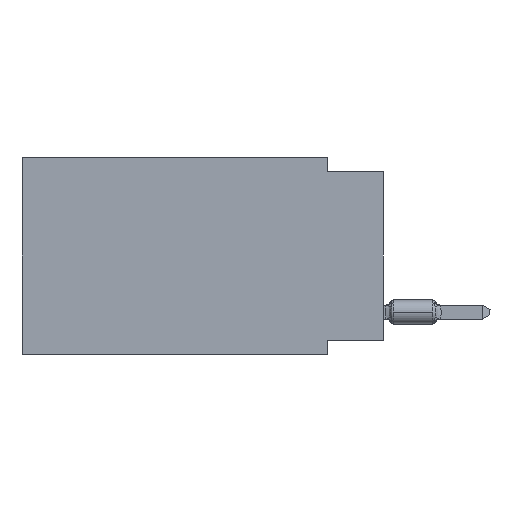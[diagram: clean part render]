
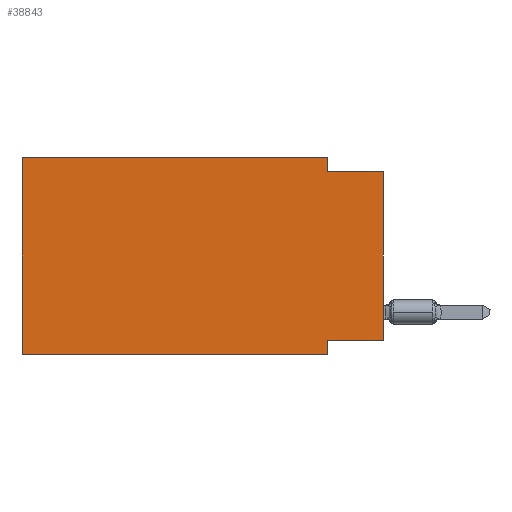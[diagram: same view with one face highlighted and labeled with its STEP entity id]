
A CAD part, left-side view. The second image highlights one B-rep face of the part: STEP entity #38843.
In plain terms, the highlighted planar face has unit normal (-1, 0, 0).
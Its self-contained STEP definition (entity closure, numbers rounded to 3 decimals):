
#959 = EDGE_CURVE ( 'NONE', #42400, #59429, #41404, .T. ) ;
#995 = CARTESIAN_POINT ( 'NONE',  ( 0., 2.54, 0. ) ) ;
#5017 = VECTOR ( 'NONE', #26155, 1000. ) ;
#5420 = VERTEX_POINT ( 'NONE', #23534 ) ;
#5710 = ORIENTED_EDGE ( 'NONE', *, *, #33910, .T. ) ;
#6240 = CARTESIAN_POINT ( 'NONE',  ( 0., 16.383, 0. ) ) ;
#8105 = VECTOR ( 'NONE', #15384, 1000. ) ;
#8938 = ORIENTED_EDGE ( 'NONE', *, *, #44442, .F. ) ;
#8968 = CARTESIAN_POINT ( 'NONE',  ( 0., 0., -8.255 ) ) ;
#9384 = LINE ( 'NONE', #24396, #17201 ) ;
#15384 = DIRECTION ( 'NONE',  ( 0., 0., -1. ) ) ;
#16372 = LINE ( 'NONE', #6240, #5017 ) ;
#17201 = VECTOR ( 'NONE', #40346, 1000. ) ;
#18650 = DIRECTION ( 'NONE',  ( 1., 0., 0. ) ) ;
#19373 = EDGE_CURVE ( 'NONE', #58460, #5420, #9384, .T. ) ;
#20087 = VECTOR ( 'NONE', #61291, 1000. ) ;
#20989 = CARTESIAN_POINT ( 'NONE',  ( 0., 2.54, -8.255 ) ) ;
#21630 = ORIENTED_EDGE ( 'NONE', *, *, #31650, .T. ) ;
#22171 = EDGE_CURVE ( 'NONE', #61417, #42400, #30371, .T. ) ;
#22909 = ORIENTED_EDGE ( 'NONE', *, *, #24747, .F. ) ;
#23534 = CARTESIAN_POINT ( 'NONE',  ( 0., 16.383, 0. ) ) ;
#24181 = VERTEX_POINT ( 'NONE', #8968 ) ;
#24396 = CARTESIAN_POINT ( 'NONE',  ( 0., 16.383, 0. ) ) ;
#24747 = EDGE_CURVE ( 'NONE', #5420, #61417, #16372, .T. ) ;
#25201 = CARTESIAN_POINT ( 'NONE',  ( 0., 16.383, -8.89 ) ) ;
#25413 = CARTESIAN_POINT ( 'NONE',  ( 0., 16.383, -8.89 ) ) ;
#25518 = DIRECTION ( 'NONE',  ( 0., -1., 0. ) ) ;
#26053 = LINE ( 'NONE', #27330, #51731 ) ;
#26155 = DIRECTION ( 'NONE',  ( 0., -1., 0. ) ) ;
#27330 = CARTESIAN_POINT ( 'NONE',  ( 0., 0., 0. ) ) ;
#27706 = CARTESIAN_POINT ( 'NONE',  ( 0., 2.54, 0. ) ) ;
#28099 = ORIENTED_EDGE ( 'NONE', *, *, #19373, .F. ) ;
#28389 = VERTEX_POINT ( 'NONE', #58267 ) ;
#28462 = DIRECTION ( 'NONE',  ( 0., 1., 0. ) ) ;
#29060 = PLANE ( 'NONE',  #57670 ) ;
#30371 = LINE ( 'NONE', #995, #8105 ) ;
#31650 = EDGE_CURVE ( 'NONE', #24181, #59429, #26053, .T. ) ;
#32051 = EDGE_LOOP ( 'NONE', ( #21630, #54140, #35988, #22909, #28099, #5710, #8938, #35703 ) ) ;
#32272 = CARTESIAN_POINT ( 'NONE',  ( 0., 0., -0.635 ) ) ;
#33348 = CARTESIAN_POINT ( 'NONE',  ( 0., 0., -8.255 ) ) ;
#33910 = EDGE_CURVE ( 'NONE', #58460, #28389, #34969, .T. ) ;
#34969 = LINE ( 'NONE', #25201, #51903 ) ;
#35703 = ORIENTED_EDGE ( 'NONE', *, *, #49704, .F. ) ;
#35988 = ORIENTED_EDGE ( 'NONE', *, *, #22171, .F. ) ;
#37371 = VECTOR ( 'NONE', #60316, 1000. ) ;
#37729 = CARTESIAN_POINT ( 'NONE',  ( 0., 0., -0.635 ) ) ;
#38843 = ADVANCED_FACE ( 'NONE', ( #58739 ), #29060, .F. ) ;
#40346 = DIRECTION ( 'NONE',  ( 0., 0., 1. ) ) ;
#41404 = LINE ( 'NONE', #32272, #20087 ) ;
#41704 = LINE ( 'NONE', #45985, #37371 ) ;
#42400 = VERTEX_POINT ( 'NONE', #47348 ) ;
#42772 = CARTESIAN_POINT ( 'NONE',  ( 0., 16.383, 0. ) ) ;
#44442 = EDGE_CURVE ( 'NONE', #60667, #28389, #41704, .T. ) ;
#45985 = CARTESIAN_POINT ( 'NONE',  ( 0., 2.54, -8.89 ) ) ;
#47348 = CARTESIAN_POINT ( 'NONE',  ( 0., 2.54, -0.635 ) ) ;
#49704 = EDGE_CURVE ( 'NONE', #24181, #60667, #53235, .T. ) ;
#51731 = VECTOR ( 'NONE', #56351, 1000. ) ;
#51903 = VECTOR ( 'NONE', #25518, 1000. ) ;
#53235 = LINE ( 'NONE', #33348, #53658 ) ;
#53658 = VECTOR ( 'NONE', #28462, 1000. ) ;
#54140 = ORIENTED_EDGE ( 'NONE', *, *, #959, .F. ) ;
#56351 = DIRECTION ( 'NONE',  ( 0., 0., 1. ) ) ;
#57670 = AXIS2_PLACEMENT_3D ( 'NONE', #42772, #18650, #62654 ) ;
#58267 = CARTESIAN_POINT ( 'NONE',  ( 0., 2.54, -8.89 ) ) ;
#58460 = VERTEX_POINT ( 'NONE', #25413 ) ;
#58739 = FACE_OUTER_BOUND ( 'NONE', #32051, .T. ) ;
#59429 = VERTEX_POINT ( 'NONE', #37729 ) ;
#60316 = DIRECTION ( 'NONE',  ( 0., 0., -1. ) ) ;
#60667 = VERTEX_POINT ( 'NONE', #20989 ) ;
#61291 = DIRECTION ( 'NONE',  ( 0., -1., 0. ) ) ;
#61417 = VERTEX_POINT ( 'NONE', #27706 ) ;
#62654 = DIRECTION ( 'NONE',  ( 0., 0., -1. ) ) ;
